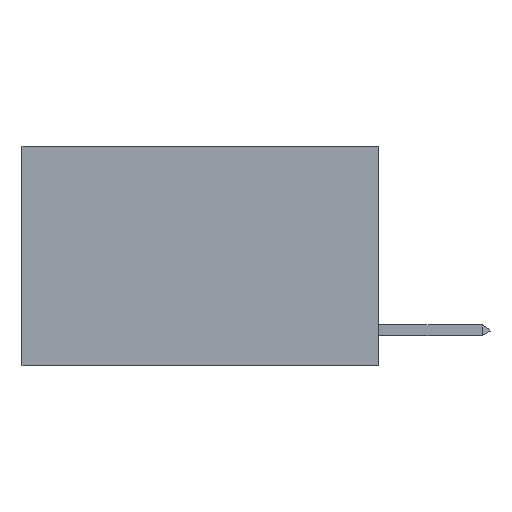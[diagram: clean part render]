
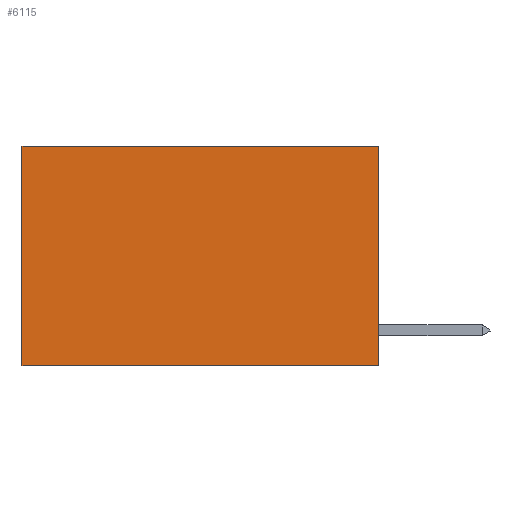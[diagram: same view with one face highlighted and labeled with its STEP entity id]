
A CAD part, left-side view. The second image highlights one B-rep face of the part: STEP entity #6115.
In plain terms, the highlighted planar face has unit normal (-1, 0, 0).
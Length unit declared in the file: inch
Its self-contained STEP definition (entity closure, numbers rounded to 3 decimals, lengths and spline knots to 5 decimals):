
#89 = AXIS2_PLACEMENT_3D ( 'NONE', #8130, #10036, #4178 ) ;
#173 = PLANE ( 'NONE',  #89 ) ;
#424 = EDGE_LOOP ( 'NONE', ( #7563, #4930, #9812, #7719 ) ) ;
#550 = EDGE_CURVE ( 'NONE', #4434, #1921, #6401, .T. ) ;
#623 = LINE ( 'NONE', #4662, #2679 ) ;
#1167 = VECTOR ( 'NONE', #7788, 39.37008 ) ;
#1921 = VERTEX_POINT ( 'NONE', #7183 ) ;
#2189 = CARTESIAN_POINT ( 'NONE',  ( 0.2625, 0., -0.37 ) ) ;
#2679 = VECTOR ( 'NONE', #5659, 39.37008 ) ;
#3177 = CARTESIAN_POINT ( 'NONE',  ( 0.2625, 0., 0. ) ) ;
#4178 = DIRECTION ( 'NONE',  ( 0., 0., -1. ) ) ;
#4182 = FACE_OUTER_BOUND ( 'NONE', #424, .T. ) ;
#4434 = VERTEX_POINT ( 'NONE', #7940 ) ;
#4463 = LINE ( 'NONE', #2189, #9378 ) ;
#4617 = VERTEX_POINT ( 'NONE', #8191 ) ;
#4662 = CARTESIAN_POINT ( 'NONE',  ( 0.2625, 0.6, 0. ) ) ;
#4759 = VECTOR ( 'NONE', #12055, 39.37008 ) ;
#4930 = ORIENTED_EDGE ( 'NONE', *, *, #7287, .F. ) ;
#5124 = CARTESIAN_POINT ( 'NONE',  ( 0.2625, 0., 0. ) ) ;
#5659 = DIRECTION ( 'NONE',  ( 0., 0., -1. ) ) ;
#6115 = ADVANCED_FACE ( 'NONE', ( #4182 ), #173, .F. ) ;
#6401 = LINE ( 'NONE', #3177, #1167 ) ;
#7183 = CARTESIAN_POINT ( 'NONE',  ( 0.2625, 0., -0.37 ) ) ;
#7287 = EDGE_CURVE ( 'NONE', #1921, #10230, #4463, .T. ) ;
#7563 = ORIENTED_EDGE ( 'NONE', *, *, #11146, .T. ) ;
#7719 = ORIENTED_EDGE ( 'NONE', *, *, #11724, .T. ) ;
#7788 = DIRECTION ( 'NONE',  ( 0., 0., -1. ) ) ;
#7940 = CARTESIAN_POINT ( 'NONE',  ( 0.2625, 0., 0. ) ) ;
#8062 = DIRECTION ( 'NONE',  ( 0., 1., 0. ) ) ;
#8085 = CARTESIAN_POINT ( 'NONE',  ( 0.2625, 0.6, -0.37 ) ) ;
#8130 = CARTESIAN_POINT ( 'NONE',  ( 0.2625, 0., 0. ) ) ;
#8191 = CARTESIAN_POINT ( 'NONE',  ( 0.2625, 0.6, 0. ) ) ;
#9378 = VECTOR ( 'NONE', #8062, 39.37008 ) ;
#9812 = ORIENTED_EDGE ( 'NONE', *, *, #550, .F. ) ;
#10036 = DIRECTION ( 'NONE',  ( 1., 0., 0. ) ) ;
#10230 = VERTEX_POINT ( 'NONE', #8085 ) ;
#11146 = EDGE_CURVE ( 'NONE', #4617, #10230, #623, .T. ) ;
#11724 = EDGE_CURVE ( 'NONE', #4434, #4617, #12604, .T. ) ;
#12055 = DIRECTION ( 'NONE',  ( 0., 1., 0. ) ) ;
#12604 = LINE ( 'NONE', #5124, #4759 ) ;
